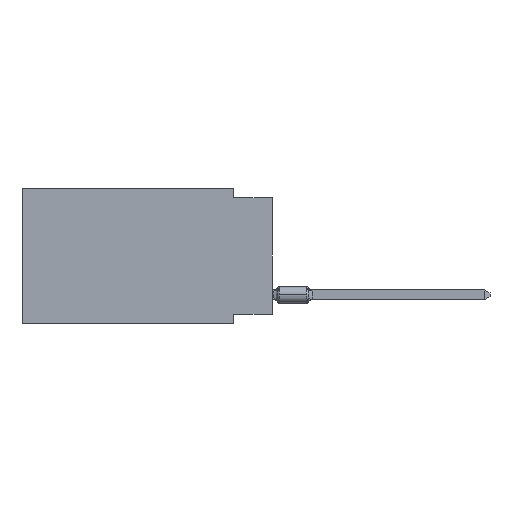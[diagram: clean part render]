
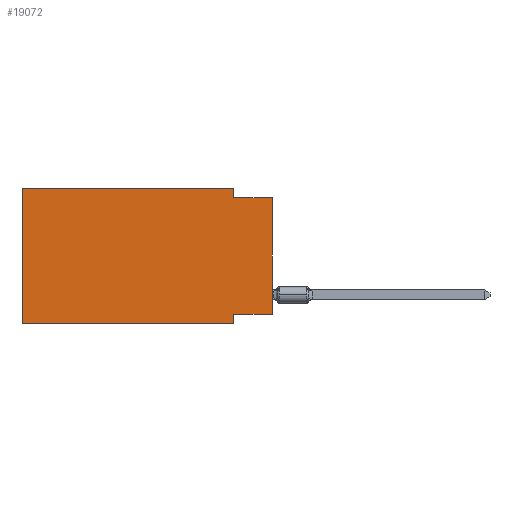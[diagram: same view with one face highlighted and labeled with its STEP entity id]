
A CAD part, left-side view. The second image highlights one B-rep face of the part: STEP entity #19072.
In plain terms, the highlighted planar face has unit normal (-1, 0, 0).
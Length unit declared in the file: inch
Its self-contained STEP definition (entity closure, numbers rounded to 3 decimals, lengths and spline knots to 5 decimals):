
#570 = LINE ( 'NONE', #17549, #16615 ) ;
#1858 = VERTEX_POINT ( 'NONE', #7100 ) ;
#2216 = CARTESIAN_POINT ( 'NONE',  ( 0., 0., -0.325 ) ) ;
#2430 = EDGE_CURVE ( 'NONE', #15242, #1858, #10869, .T. ) ;
#3230 = VERTEX_POINT ( 'NONE', #2216 ) ;
#3857 = LINE ( 'NONE', #9904, #18239 ) ;
#3946 = EDGE_CURVE ( 'NONE', #3230, #5988, #9084, .T. ) ;
#3973 = ORIENTED_EDGE ( 'NONE', *, *, #18003, .F. ) ;
#4295 = ORIENTED_EDGE ( 'NONE', *, *, #2430, .F. ) ;
#4626 = VERTEX_POINT ( 'NONE', #11444 ) ;
#5114 = EDGE_CURVE ( 'NONE', #1858, #5988, #14794, .T. ) ;
#5252 = DIRECTION ( 'NONE',  ( 0., -1., 0. ) ) ;
#5518 = ORIENTED_EDGE ( 'NONE', *, *, #11384, .F. ) ;
#5988 = VERTEX_POINT ( 'NONE', #15312 ) ;
#6011 = LINE ( 'NONE', #12185, #6345 ) ;
#6345 = VECTOR ( 'NONE', #17953, 39.37008 ) ;
#6625 = CARTESIAN_POINT ( 'NONE',  ( 0., 0.1, -0.35 ) ) ;
#6796 = DIRECTION ( 'NONE',  ( 0., -1., 0. ) ) ;
#6812 = ORIENTED_EDGE ( 'NONE', *, *, #10208, .T. ) ;
#7100 = CARTESIAN_POINT ( 'NONE',  ( 0., 0.1, -0.025 ) ) ;
#7163 = VECTOR ( 'NONE', #15257, 39.37008 ) ;
#7215 = CARTESIAN_POINT ( 'NONE',  ( 0., 0., -0.025 ) ) ;
#8446 = AXIS2_PLACEMENT_3D ( 'NONE', #13148, #13249, #19312 ) ;
#8859 = CARTESIAN_POINT ( 'NONE',  ( 0., 0.645, -0.35 ) ) ;
#8870 = ORIENTED_EDGE ( 'NONE', *, *, #3946, .T. ) ;
#9084 = LINE ( 'NONE', #9183, #7163 ) ;
#9183 = CARTESIAN_POINT ( 'NONE',  ( 0., 0., 0. ) ) ;
#9904 = CARTESIAN_POINT ( 'NONE',  ( 0., 0.645, 0. ) ) ;
#9911 = DIRECTION ( 'NONE',  ( 0., 1., 0. ) ) ;
#10208 = EDGE_CURVE ( 'NONE', #14547, #19259, #6011, .T. ) ;
#10391 = VECTOR ( 'NONE', #5252, 39.37008 ) ;
#10701 = ORIENTED_EDGE ( 'NONE', *, *, #15672, .F. ) ;
#10869 = LINE ( 'NONE', #18129, #12544 ) ;
#11028 = DIRECTION ( 'NONE',  ( 0., 0., -1. ) ) ;
#11226 = CARTESIAN_POINT ( 'NONE',  ( 0., 0.1, 0. ) ) ;
#11361 = PLANE ( 'NONE',  #8446 ) ;
#11384 = EDGE_CURVE ( 'NONE', #17990, #19259, #15975, .T. ) ;
#11444 = CARTESIAN_POINT ( 'NONE',  ( 0., 0.645, 0. ) ) ;
#12050 = ORIENTED_EDGE ( 'NONE', *, *, #5114, .F. ) ;
#12185 = CARTESIAN_POINT ( 'NONE',  ( 0., 0.645, -0.35 ) ) ;
#12423 = CARTESIAN_POINT ( 'NONE',  ( 0., 0.1, -0.325 ) ) ;
#12544 = VECTOR ( 'NONE', #13760, 39.37008 ) ;
#13012 = CARTESIAN_POINT ( 'NONE',  ( 0., 0., -0.325 ) ) ;
#13148 = CARTESIAN_POINT ( 'NONE',  ( 0., 0.645, 0. ) ) ;
#13249 = DIRECTION ( 'NONE',  ( 1., 0., 0. ) ) ;
#13343 = CARTESIAN_POINT ( 'NONE',  ( 0., 0.1, -0.35 ) ) ;
#13460 = EDGE_LOOP ( 'NONE', ( #8870, #12050, #4295, #19353, #10701, #6812, #5518, #3973 ) ) ;
#13760 = DIRECTION ( 'NONE',  ( 0., 0., -1. ) ) ;
#14178 = EDGE_CURVE ( 'NONE', #4626, #15242, #570, .T. ) ;
#14547 = VERTEX_POINT ( 'NONE', #8859 ) ;
#14794 = LINE ( 'NONE', #7215, #10391 ) ;
#15242 = VERTEX_POINT ( 'NONE', #11226 ) ;
#15257 = DIRECTION ( 'NONE',  ( 0., 0., 1. ) ) ;
#15312 = CARTESIAN_POINT ( 'NONE',  ( 0., 0., -0.025 ) ) ;
#15672 = EDGE_CURVE ( 'NONE', #14547, #4626, #3857, .T. ) ;
#15759 = VECTOR ( 'NONE', #9911, 39.37008 ) ;
#15975 = LINE ( 'NONE', #6625, #16873 ) ;
#16615 = VECTOR ( 'NONE', #6796, 39.37008 ) ;
#16873 = VECTOR ( 'NONE', #11028, 39.37008 ) ;
#17263 = DIRECTION ( 'NONE',  ( 0., 0., 1. ) ) ;
#17549 = CARTESIAN_POINT ( 'NONE',  ( 0., 0.645, 0. ) ) ;
#17953 = DIRECTION ( 'NONE',  ( 0., -1., 0. ) ) ;
#17990 = VERTEX_POINT ( 'NONE', #12423 ) ;
#18003 = EDGE_CURVE ( 'NONE', #3230, #17990, #19067, .T. ) ;
#18129 = CARTESIAN_POINT ( 'NONE',  ( 0., 0.1, 0. ) ) ;
#18239 = VECTOR ( 'NONE', #17263, 39.37008 ) ;
#19067 = LINE ( 'NONE', #13012, #15759 ) ;
#19072 = ADVANCED_FACE ( 'NONE', ( #19207 ), #11361, .F. ) ;
#19207 = FACE_OUTER_BOUND ( 'NONE', #13460, .T. ) ;
#19259 = VERTEX_POINT ( 'NONE', #13343 ) ;
#19312 = DIRECTION ( 'NONE',  ( 0., 0., -1. ) ) ;
#19353 = ORIENTED_EDGE ( 'NONE', *, *, #14178, .F. ) ;
